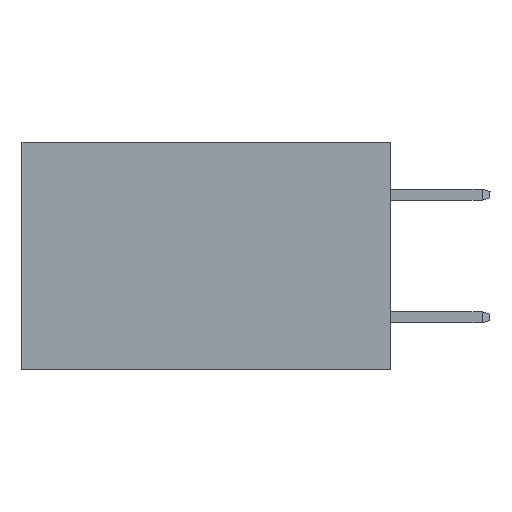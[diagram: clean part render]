
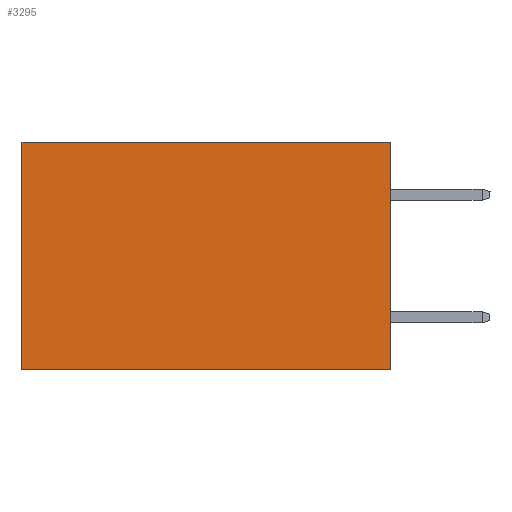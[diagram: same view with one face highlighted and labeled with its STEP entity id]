
A CAD part, left-side view. The second image highlights one B-rep face of the part: STEP entity #3295.
In plain terms, the highlighted planar face has unit normal (-1, 0, 0).
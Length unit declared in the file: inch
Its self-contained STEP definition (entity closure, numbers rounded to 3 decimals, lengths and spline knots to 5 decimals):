
#22 = ORIENTED_EDGE ( 'NONE', *, *, #5180, .F. ) ;
#48 = VECTOR ( 'NONE', #7225, 39.37008 ) ;
#169 = VECTOR ( 'NONE', #5921, 39.37008 ) ;
#521 = VERTEX_POINT ( 'NONE', #8433 ) ;
#525 = VECTOR ( 'NONE', #4371, 39.37008 ) ;
#585 = VERTEX_POINT ( 'NONE', #6985 ) ;
#1004 = LINE ( 'NONE', #4340, #525 ) ;
#1277 = CARTESIAN_POINT ( 'NONE',  ( 0.2875, 0., -0.37 ) ) ;
#1618 = VECTOR ( 'NONE', #9711, 39.37008 ) ;
#1783 = EDGE_CURVE ( 'NONE', #585, #9891, #4608, .T. ) ;
#1887 = DIRECTION ( 'NONE',  ( 1., 0., 0. ) ) ;
#2443 = FACE_OUTER_BOUND ( 'NONE', #5916, .T. ) ;
#3295 = ADVANCED_FACE ( 'NONE', ( #2443 ), #6532, .F. ) ;
#3311 = ORIENTED_EDGE ( 'NONE', *, *, #9865, .F. ) ;
#3360 = ORIENTED_EDGE ( 'NONE', *, *, #9812, .T. ) ;
#4260 = CARTESIAN_POINT ( 'NONE',  ( 0.2875, 0.6, 0. ) ) ;
#4340 = CARTESIAN_POINT ( 'NONE',  ( 0.2875, 0., -0.37 ) ) ;
#4371 = DIRECTION ( 'NONE',  ( 0., 1., 0. ) ) ;
#4608 = LINE ( 'NONE', #5223, #169 ) ;
#4944 = DIRECTION ( 'NONE',  ( 0., 0., -1. ) ) ;
#5180 = EDGE_CURVE ( 'NONE', #585, #6655, #7442, .T. ) ;
#5223 = CARTESIAN_POINT ( 'NONE',  ( 0.2875, 0., 0. ) ) ;
#5916 = EDGE_LOOP ( 'NONE', ( #3360, #3311, #22, #7118 ) ) ;
#5921 = DIRECTION ( 'NONE',  ( 0., 1., 0. ) ) ;
#6532 = PLANE ( 'NONE',  #9889 ) ;
#6655 = VERTEX_POINT ( 'NONE', #1277 ) ;
#6985 = CARTESIAN_POINT ( 'NONE',  ( 0.2875, 0., 0. ) ) ;
#7118 = ORIENTED_EDGE ( 'NONE', *, *, #1783, .T. ) ;
#7225 = DIRECTION ( 'NONE',  ( 0., 0., -1. ) ) ;
#7442 = LINE ( 'NONE', #8694, #48 ) ;
#8085 = CARTESIAN_POINT ( 'NONE',  ( 0.2875, 0., 0. ) ) ;
#8433 = CARTESIAN_POINT ( 'NONE',  ( 0.2875, 0.6, -0.37 ) ) ;
#8542 = CARTESIAN_POINT ( 'NONE',  ( 0.2875, 0.6, 0. ) ) ;
#8694 = CARTESIAN_POINT ( 'NONE',  ( 0.2875, 0., 0. ) ) ;
#9711 = DIRECTION ( 'NONE',  ( 0., 0., -1. ) ) ;
#9741 = LINE ( 'NONE', #4260, #1618 ) ;
#9812 = EDGE_CURVE ( 'NONE', #9891, #521, #9741, .T. ) ;
#9865 = EDGE_CURVE ( 'NONE', #6655, #521, #1004, .T. ) ;
#9889 = AXIS2_PLACEMENT_3D ( 'NONE', #8085, #1887, #4944 ) ;
#9891 = VERTEX_POINT ( 'NONE', #8542 ) ;
